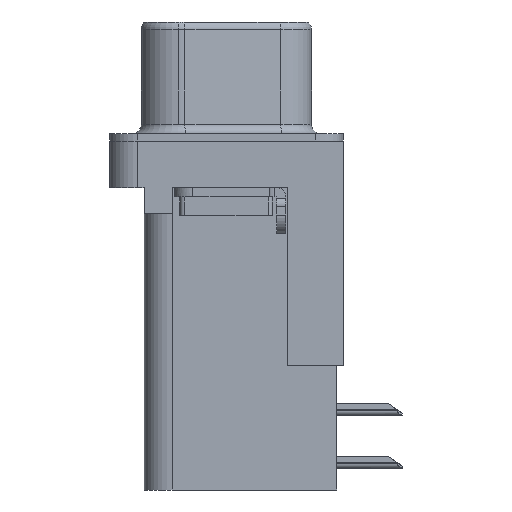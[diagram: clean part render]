
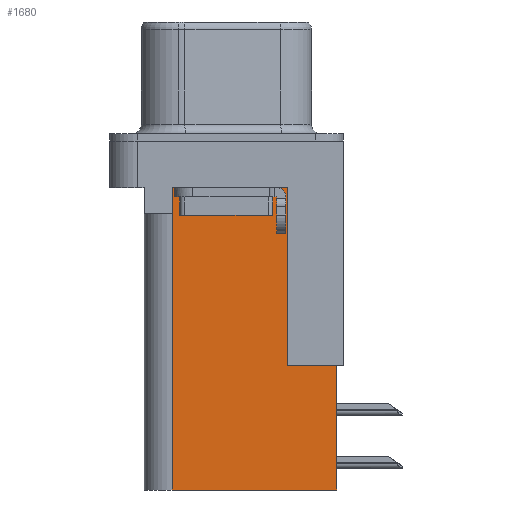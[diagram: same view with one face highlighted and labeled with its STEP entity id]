
A CAD part, left-side view. The second image highlights one B-rep face of the part: STEP entity #1680.
In plain terms, the highlighted planar face has unit normal (-1, 0, 0).
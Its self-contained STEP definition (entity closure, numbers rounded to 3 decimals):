
#73 = CARTESIAN_POINT ( 'NONE',  ( 3.7, -5.925, -2. ) ) ;
#502 = AXIS2_PLACEMENT_3D ( 'NONE', #5855, #6598, #13846 ) ;
#586 = CARTESIAN_POINT ( 'NONE',  ( 3.7, -6.295, -12.05 ) ) ;
#605 = FACE_OUTER_BOUND ( 'NONE', #1294, .T. ) ;
#946 = LINE ( 'NONE', #8630, #13029 ) ;
#1293 = CARTESIAN_POINT ( 'NONE',  ( 3.7, -3.295, -2.5 ) ) ;
#1294 = EDGE_LOOP ( 'NONE', ( #14734, #4495, #3775, #13077, #18323, #4612, #7546, #18153 ) ) ;
#1300 = VERTEX_POINT ( 'NONE', #15197 ) ;
#1680 = ADVANCED_FACE ( 'NONE', ( #605 ), #3648, .F. ) ;
#2065 = VECTOR ( 'NONE', #14107, 1000. ) ;
#2119 = CARTESIAN_POINT ( 'NONE',  ( 3.7, -3.295, -18.76 ) ) ;
#2421 = EDGE_CURVE ( 'NONE', #11301, #12568, #13676, .T. ) ;
#2766 = EDGE_CURVE ( 'NONE', #12568, #10871, #12666, .T. ) ;
#3171 = EDGE_CURVE ( 'NONE', #10871, #1300, #18785, .T. ) ;
#3442 = VECTOR ( 'NONE', #3752, 1000. ) ;
#3633 = CARTESIAN_POINT ( 'NONE',  ( 3.7, 2.895, -3.9 ) ) ;
#3648 = PLANE ( 'NONE',  #502 ) ;
#3662 = DIRECTION ( 'NONE',  ( 0., 1., 0. ) ) ;
#3752 = DIRECTION ( 'NONE',  ( 0., 1., 0. ) ) ;
#3775 = ORIENTED_EDGE ( 'NONE', *, *, #3171, .T. ) ;
#4495 = ORIENTED_EDGE ( 'NONE', *, *, #2766, .T. ) ;
#4612 = ORIENTED_EDGE ( 'NONE', *, *, #8666, .F. ) ;
#4753 = CARTESIAN_POINT ( 'NONE',  ( 3.7, -5.925, -12.05 ) ) ;
#4854 = VECTOR ( 'NONE', #5041, 1000. ) ;
#5041 = DIRECTION ( 'NONE',  ( 0., 0., -1. ) ) ;
#5073 = CARTESIAN_POINT ( 'NONE',  ( 3.7, -3.295, -12.05 ) ) ;
#5489 = EDGE_CURVE ( 'NONE', #14548, #1300, #17106, .T. ) ;
#5715 = VECTOR ( 'NONE', #14728, 1000. ) ;
#5855 = CARTESIAN_POINT ( 'NONE',  ( 3.7, -3.295, -18.76 ) ) ;
#6598 = DIRECTION ( 'NONE',  ( 1., 0., 0. ) ) ;
#7546 = ORIENTED_EDGE ( 'NONE', *, *, #19333, .T. ) ;
#7725 = VECTOR ( 'NONE', #18931, 1000. ) ;
#8105 = VERTEX_POINT ( 'NONE', #5073 ) ;
#8518 = CARTESIAN_POINT ( 'NONE',  ( 3.7, -3.295, -2.5 ) ) ;
#8630 = CARTESIAN_POINT ( 'NONE',  ( 3.7, -3.295, -18.76 ) ) ;
#8659 = CARTESIAN_POINT ( 'NONE',  ( 3.7, -5.925, -18.76 ) ) ;
#8666 = EDGE_CURVE ( 'NONE', #18607, #13155, #16527, .T. ) ;
#9858 = LINE ( 'NONE', #586, #5715 ) ;
#10871 = VERTEX_POINT ( 'NONE', #12190 ) ;
#11301 = VERTEX_POINT ( 'NONE', #8518 ) ;
#11829 = CARTESIAN_POINT ( 'NONE',  ( 3.7, 2.925, -18.76 ) ) ;
#12190 = CARTESIAN_POINT ( 'NONE',  ( 3.7, 2.895, -3.9 ) ) ;
#12568 = VERTEX_POINT ( 'NONE', #14909 ) ;
#12666 = LINE ( 'NONE', #3633, #4854 ) ;
#12811 = DIRECTION ( 'NONE',  ( 0., 0., 1. ) ) ;
#13029 = VECTOR ( 'NONE', #14933, 1000. ) ;
#13077 = ORIENTED_EDGE ( 'NONE', *, *, #5489, .F. ) ;
#13155 = VERTEX_POINT ( 'NONE', #8659 ) ;
#13307 = CARTESIAN_POINT ( 'NONE',  ( 3.7, 2.925, -18.76 ) ) ;
#13676 = LINE ( 'NONE', #1293, #17321 ) ;
#13846 = DIRECTION ( 'NONE',  ( 0., 1., 0. ) ) ;
#14107 = DIRECTION ( 'NONE',  ( 0., 1., 0. ) ) ;
#14548 = VERTEX_POINT ( 'NONE', #11829 ) ;
#14728 = DIRECTION ( 'NONE',  ( 0., 1., 0. ) ) ;
#14734 = ORIENTED_EDGE ( 'NONE', *, *, #2421, .T. ) ;
#14909 = CARTESIAN_POINT ( 'NONE',  ( 3.7, 2.895, -2.5 ) ) ;
#14933 = DIRECTION ( 'NONE',  ( 0., 0., 1. ) ) ;
#15197 = CARTESIAN_POINT ( 'NONE',  ( 3.7, 2.925, -3.9 ) ) ;
#15660 = VECTOR ( 'NONE', #12811, 1000. ) ;
#15940 = LINE ( 'NONE', #2119, #3442 ) ;
#16204 = CARTESIAN_POINT ( 'NONE',  ( 3.7, 0., -3.9 ) ) ;
#16527 = LINE ( 'NONE', #73, #7725 ) ;
#17106 = LINE ( 'NONE', #13307, #15660 ) ;
#17321 = VECTOR ( 'NONE', #3662, 1000. ) ;
#18153 = ORIENTED_EDGE ( 'NONE', *, *, #19401, .T. ) ;
#18323 = ORIENTED_EDGE ( 'NONE', *, *, #19669, .F. ) ;
#18607 = VERTEX_POINT ( 'NONE', #4753 ) ;
#18785 = LINE ( 'NONE', #16204, #2065 ) ;
#18931 = DIRECTION ( 'NONE',  ( 0., 0., -1. ) ) ;
#19333 = EDGE_CURVE ( 'NONE', #18607, #8105, #9858, .T. ) ;
#19401 = EDGE_CURVE ( 'NONE', #8105, #11301, #946, .T. ) ;
#19669 = EDGE_CURVE ( 'NONE', #13155, #14548, #15940, .T. ) ;
